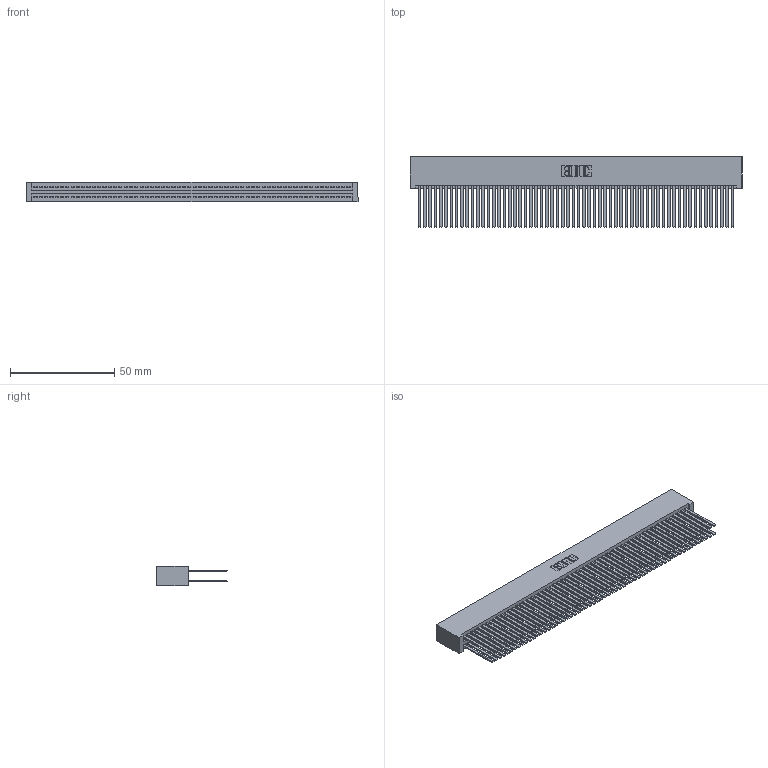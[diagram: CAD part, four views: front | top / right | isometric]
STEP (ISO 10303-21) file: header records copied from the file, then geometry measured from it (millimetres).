
FILE_DESCRIPTION (( 'STEP AP203' ), '1' );
FILE_NAME ('845-120-544-201.STEP', '2018-11-21T04:37:24', ( '' ), ( '' ), 'SwSTEP 2.0', 'SolidWorks 2016', '' );
FILE_SCHEMA (( 'CONFIG_CONTROL_DESIGN' ));
Length unit declared in the file: inch
Products named in the file (3): 845 Part_No Mounting Lugs; 345-292-001_345-293-144; 845-120-544-201
Assembly tree (121 placements, depth 2):
  845-120-544-201
    845 Part_No Mounting Lugs
    345-292-001_345-293-144  x120
Bounding box: 159 x 33.96 x 9.4 mm (x, y, z)
Volume: 17911 mm3; surface area: 32057.6 mm2
Topology: 121 solids, 121 shells, 5398 faces, 16037 edges, 10530 vertices
Faces by surface type: plane 3556, cylinder 1842
Entity records: 44193 total; most frequent: CARTESIAN_POINT 7388, ORIENTED_EDGE 7322, DIRECTION 6485, EDGE_CURVE 3661, LINE 3301, VECTOR 3301, VERTEX_POINT 2438, AXIS2_PLACEMENT_3D 1592
